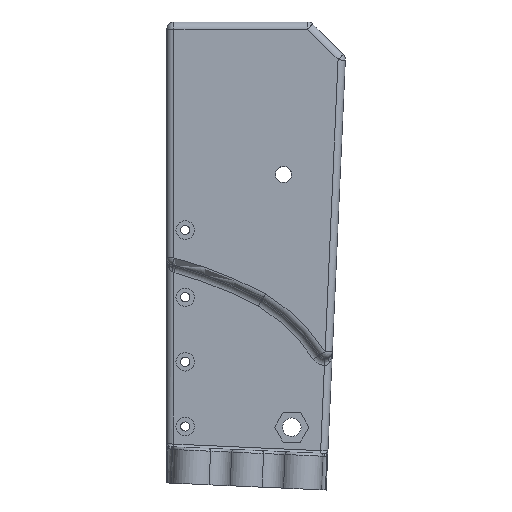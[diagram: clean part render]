
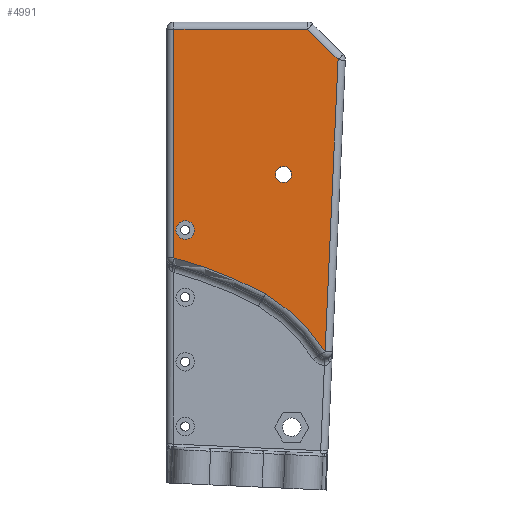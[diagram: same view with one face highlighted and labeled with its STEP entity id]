
A CAD part, left-side view. The second image highlights one B-rep face of the part: STEP entity #4991.
In plain terms, the highlighted planar face has unit normal (-1, 0, 0).
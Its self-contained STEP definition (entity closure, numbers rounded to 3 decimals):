
#135=FACE_BOUND('',#623,.T.);
#136=FACE_BOUND('',#624,.T.);
#208=PLANE('',#5323);
#326=FACE_OUTER_BOUND('',#622,.T.);
#622=EDGE_LOOP('',(#3495,#3496,#3497,#3498,#3499,#3500));
#623=EDGE_LOOP('',(#3501));
#624=EDGE_LOOP('',(#3502,#3503));
#948=CIRCLE('',#5324,122.);
#949=CIRCLE('',#5325,52.);
#950=CIRCLE('',#5326,2.25);
#951=CIRCLE('',#5327,2.54);
#952=CIRCLE('',#5328,2.54);
#1448=LINE('',#25656,#1730);
#1449=LINE('',#25663,#1731);
#1450=LINE('',#25665,#1732);
#1451=LINE('',#25670,#1733);
#1730=VECTOR('',#5945,10.);
#1731=VECTOR('',#5954,10.);
#1732=VECTOR('',#5955,10.);
#1733=VECTOR('',#5960,10.);
#2122=VERTEX_POINT('',#25648);
#2123=VERTEX_POINT('',#25652);
#2126=VERTEX_POINT('',#25662);
#2127=VERTEX_POINT('',#25664);
#2128=VERTEX_POINT('',#25666);
#2129=VERTEX_POINT('',#25668);
#2130=VERTEX_POINT('',#25671);
#2131=VERTEX_POINT('',#25673);
#2132=VERTEX_POINT('',#25674);
#2667=EDGE_CURVE('',#2122,#2123,#1448,.T.);
#2670=EDGE_CURVE('',#2126,#2122,#1449,.T.);
#2671=EDGE_CURVE('',#2127,#2126,#1450,.T.);
#2672=EDGE_CURVE('',#2128,#2127,#948,.T.);
#2673=EDGE_CURVE('',#2129,#2128,#949,.T.);
#2674=EDGE_CURVE('',#2123,#2129,#1451,.T.);
#2675=EDGE_CURVE('',#2130,#2130,#950,.T.);
#2676=EDGE_CURVE('',#2131,#2132,#951,.T.);
#2677=EDGE_CURVE('',#2132,#2131,#952,.T.);
#3495=ORIENTED_EDGE('',*,*,#2667,.F.);
#3496=ORIENTED_EDGE('',*,*,#2670,.F.);
#3497=ORIENTED_EDGE('',*,*,#2671,.F.);
#3498=ORIENTED_EDGE('',*,*,#2672,.F.);
#3499=ORIENTED_EDGE('',*,*,#2673,.F.);
#3500=ORIENTED_EDGE('',*,*,#2674,.F.);
#3501=ORIENTED_EDGE('',*,*,#2675,.T.);
#3502=ORIENTED_EDGE('',*,*,#2676,.F.);
#3503=ORIENTED_EDGE('',*,*,#2677,.F.);
#4991=ADVANCED_FACE('',(#326,#135,#136),#208,.F.);
#5323=AXIS2_PLACEMENT_3D('',#25661,#5952,#5953);
#5324=AXIS2_PLACEMENT_3D('',#25667,#5956,#5957);
#5325=AXIS2_PLACEMENT_3D('',#25669,#5958,#5959);
#5326=AXIS2_PLACEMENT_3D('',#25672,#5961,#5962);
#5327=AXIS2_PLACEMENT_3D('',#25675,#5963,#5964);
#5328=AXIS2_PLACEMENT_3D('',#25676,#5965,#5966);
#5945=DIRECTION('',(0.,-0.707,-0.707));
#5952=DIRECTION('center_axis',(1.,0.,0.));
#5953=DIRECTION('ref_axis',(0.,0.,-1.));
#5954=DIRECTION('',(0.,-1.,0.));
#5955=DIRECTION('',(0.,0.,1.));
#5956=DIRECTION('center_axis',(-1.,0.,0.));
#5957=DIRECTION('ref_axis',(0.,-0.36,0.933));
#5958=DIRECTION('center_axis',(-1.,0.,0.));
#5959=DIRECTION('ref_axis',(0.,-0.742,0.67));
#5960=DIRECTION('',(0.,0.044,-0.999));
#5961=DIRECTION('center_axis',(1.,0.,0.));
#5962=DIRECTION('ref_axis',(0.,0.,1.));
#5963=DIRECTION('center_axis',(-1.,0.,0.));
#5964=DIRECTION('ref_axis',(0.,0.,-1.));
#5965=DIRECTION('center_axis',(-1.,0.,0.));
#5966=DIRECTION('ref_axis',(0.,0.,-1.));
#25648=CARTESIAN_POINT('',(-30.1,-38.819,283.));
#25652=CARTESIAN_POINT('',(-30.1,-47.232,274.587));
#25656=CARTESIAN_POINT('',(-30.1,-48.759,273.06));
#25661=CARTESIAN_POINT('Origin',(-30.1,-24.313,243.358));
#25662=CARTESIAN_POINT('',(-30.1,-2.086,283.));
#25663=CARTESIAN_POINT('',(-30.1,-21.538,283.));
#25664=CARTESIAN_POINT('',(-30.1,-2.086,220.116));
#25665=CARTESIAN_POINT('',(-30.1,-2.086,121.679));
#25666=CARTESIAN_POINT('',(-30.1,-27.248,210.212));
#25667=CARTESIAN_POINT('Origin',(-30.1,29.741,102.34));
#25668=CARTESIAN_POINT('',(-30.1,-43.66,194.375));
#25669=CARTESIAN_POINT('Origin',(-30.1,-0.224,165.785));
#25670=CARTESIAN_POINT('',(-30.1,-41.669,149.68));
#25671=CARTESIAN_POINT('',(-30.1,-32.23,240.784));
#25672=CARTESIAN_POINT('Origin',(-30.1,-32.23,243.034));
#25673=CARTESIAN_POINT('',(-30.1,-5.186,230.306));
#25674=CARTESIAN_POINT('',(-30.1,-5.186,225.226));
#25675=CARTESIAN_POINT('Origin',(-30.1,-5.186,227.766));
#25676=CARTESIAN_POINT('Origin',(-30.1,-5.186,227.766));
